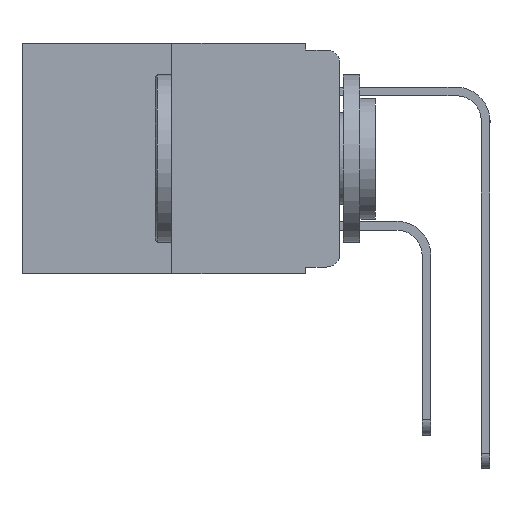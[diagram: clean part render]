
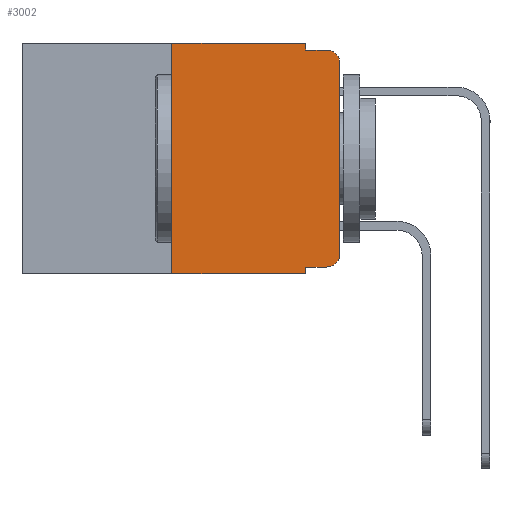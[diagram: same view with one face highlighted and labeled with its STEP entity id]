
A CAD part, left-side view. The second image highlights one B-rep face of the part: STEP entity #3002.
In plain terms, the highlighted planar face has unit normal (-1, 0, 0).
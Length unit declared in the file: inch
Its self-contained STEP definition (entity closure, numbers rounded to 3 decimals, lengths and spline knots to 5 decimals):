
#297 = EDGE_CURVE ( 'NONE', #541, #1149, #525, .T. ) ;
#336 = LINE ( 'NONE', #15332, #4701 ) ;
#396 = ORIENTED_EDGE ( 'NONE', *, *, #9617, .F. ) ;
#525 = LINE ( 'NONE', #19339, #12760 ) ;
#541 = VERTEX_POINT ( 'NONE', #13441 ) ;
#1149 = VERTEX_POINT ( 'NONE', #13604 ) ;
#1391 = VERTEX_POINT ( 'NONE', #6927 ) ;
#1458 = ORIENTED_EDGE ( 'NONE', *, *, #6786, .F. ) ;
#1470 = VERTEX_POINT ( 'NONE', #7637 ) ;
#1558 = LINE ( 'NONE', #17015, #4329 ) ;
#1567 = VERTEX_POINT ( 'NONE', #2991 ) ;
#1580 = DIRECTION ( 'NONE',  ( 0., 0., -1. ) ) ;
#1585 = DIRECTION ( 'NONE',  ( -1., 0., 0. ) ) ;
#1731 = LINE ( 'NONE', #12327, #9806 ) ;
#1735 = CARTESIAN_POINT ( 'NONE',  ( 0., 0.02, -0.03 ) ) ;
#2250 = CARTESIAN_POINT ( 'NONE',  ( 0., 0.051, -0.01 ) ) ;
#2991 = CARTESIAN_POINT ( 'NONE',  ( 0., 0.051, -0.343 ) ) ;
#3002 = ADVANCED_FACE ( 'NONE', ( #5109 ), #8063, .F. ) ;
#3426 = CARTESIAN_POINT ( 'NONE',  ( 0., 0.02, -0.313 ) ) ;
#3467 = ORIENTED_EDGE ( 'NONE', *, *, #17407, .F. ) ;
#3542 = CARTESIAN_POINT ( 'NONE',  ( 0., 0.02, -0.01 ) ) ;
#3921 = EDGE_CURVE ( 'NONE', #1391, #6474, #5566, .T. ) ;
#4329 = VECTOR ( 'NONE', #20122, 39.37008 ) ;
#4465 = CARTESIAN_POINT ( 'NONE',  ( 0., 0.02, -0.333 ) ) ;
#4498 = ORIENTED_EDGE ( 'NONE', *, *, #11927, .F. ) ;
#4673 = CIRCLE ( 'NONE', #9101, 0.02 ) ;
#4701 = VECTOR ( 'NONE', #6015, 39.37008 ) ;
#4958 = VECTOR ( 'NONE', #9388, 39.37008 ) ;
#5074 = DIRECTION ( 'NONE',  ( 0., 0., -1. ) ) ;
#5109 = FACE_OUTER_BOUND ( 'NONE', #13820, .T. ) ;
#5357 = CARTESIAN_POINT ( 'NONE',  ( 0., 0., -0.313 ) ) ;
#5566 = CIRCLE ( 'NONE', #9823, 0.02 ) ;
#5815 = VERTEX_POINT ( 'NONE', #14480 ) ;
#6015 = DIRECTION ( 'NONE',  ( 0., 0., -1. ) ) ;
#6028 = ORIENTED_EDGE ( 'NONE', *, *, #18913, .T. ) ;
#6474 = VERTEX_POINT ( 'NONE', #3542 ) ;
#6740 = DIRECTION ( 'NONE',  ( 0., 0., -1. ) ) ;
#6761 = DIRECTION ( 'NONE',  ( 1., 0., 0. ) ) ;
#6786 = EDGE_CURVE ( 'NONE', #1149, #5815, #8750, .T. ) ;
#6927 = CARTESIAN_POINT ( 'NONE',  ( 0., 0., -0.03 ) ) ;
#7637 = CARTESIAN_POINT ( 'NONE',  ( 0., 0.051, -0.333 ) ) ;
#7797 = ORIENTED_EDGE ( 'NONE', *, *, #12364, .T. ) ;
#7957 = CARTESIAN_POINT ( 'NONE',  ( 0., 0.473, 0. ) ) ;
#8063 = PLANE ( 'NONE',  #14039 ) ;
#8750 = LINE ( 'NONE', #9354, #4958 ) ;
#9101 = AXIS2_PLACEMENT_3D ( 'NONE', #3426, #14441, #5074 ) ;
#9354 = CARTESIAN_POINT ( 'NONE',  ( 0., 0.051, 0. ) ) ;
#9388 = DIRECTION ( 'NONE',  ( 0., 0., -1. ) ) ;
#9617 = EDGE_CURVE ( 'NONE', #5815, #6474, #14612, .T. ) ;
#9806 = VECTOR ( 'NONE', #13849, 39.37008 ) ;
#9823 = AXIS2_PLACEMENT_3D ( 'NONE', #1735, #1585, #1580 ) ;
#10190 = CARTESIAN_POINT ( 'NONE',  ( 0., 0.473, -0.343 ) ) ;
#10750 = ORIENTED_EDGE ( 'NONE', *, *, #15227, .T. ) ;
#11448 = VERTEX_POINT ( 'NONE', #4465 ) ;
#11927 = EDGE_CURVE ( 'NONE', #1470, #1567, #336, .T. ) ;
#12162 = ORIENTED_EDGE ( 'NONE', *, *, #14460, .T. ) ;
#12327 = CARTESIAN_POINT ( 'NONE',  ( 0., 0.051, -0.333 ) ) ;
#12335 = VERTEX_POINT ( 'NONE', #5357 ) ;
#12364 = EDGE_CURVE ( 'NONE', #18780, #1567, #17575, .T. ) ;
#12677 = DIRECTION ( 'NONE',  ( 0., 0., 1. ) ) ;
#12760 = VECTOR ( 'NONE', #19252, 39.37008 ) ;
#13189 = VECTOR ( 'NONE', #17928, 39.37008 ) ;
#13441 = CARTESIAN_POINT ( 'NONE',  ( 0., 0.25, 0. ) ) ;
#13525 = CARTESIAN_POINT ( 'NONE',  ( 0., 0.25, -0.343 ) ) ;
#13604 = CARTESIAN_POINT ( 'NONE',  ( 0., 0.051, 0. ) ) ;
#13820 = EDGE_LOOP ( 'NONE', ( #12162, #16705, #396, #1458, #19065, #3467, #7797, #4498, #6028, #10750 ) ) ;
#13849 = DIRECTION ( 'NONE',  ( 0., -1., 0. ) ) ;
#14039 = AXIS2_PLACEMENT_3D ( 'NONE', #7957, #6761, #6740 ) ;
#14441 = DIRECTION ( 'NONE',  ( -1., 0., 0. ) ) ;
#14460 = EDGE_CURVE ( 'NONE', #12335, #1391, #18706, .T. ) ;
#14480 = CARTESIAN_POINT ( 'NONE',  ( 0., 0.051, -0.01 ) ) ;
#14612 = LINE ( 'NONE', #2250, #13189 ) ;
#14660 = VECTOR ( 'NONE', #12677, 39.37008 ) ;
#14781 = DIRECTION ( 'NONE',  ( 0., -1., 0. ) ) ;
#15227 = EDGE_CURVE ( 'NONE', #11448, #12335, #4673, .T. ) ;
#15332 = CARTESIAN_POINT ( 'NONE',  ( 0., 0.051, 0. ) ) ;
#16633 = VECTOR ( 'NONE', #14781, 39.37008 ) ;
#16705 = ORIENTED_EDGE ( 'NONE', *, *, #3921, .T. ) ;
#17015 = CARTESIAN_POINT ( 'NONE',  ( 0., 0.25, 0. ) ) ;
#17407 = EDGE_CURVE ( 'NONE', #18780, #541, #1558, .T. ) ;
#17575 = LINE ( 'NONE', #10190, #16633 ) ;
#17928 = DIRECTION ( 'NONE',  ( 0., -1., 0. ) ) ;
#18706 = LINE ( 'NONE', #18731, #14660 ) ;
#18731 = CARTESIAN_POINT ( 'NONE',  ( 0., 0., 0. ) ) ;
#18780 = VERTEX_POINT ( 'NONE', #13525 ) ;
#18913 = EDGE_CURVE ( 'NONE', #1470, #11448, #1731, .T. ) ;
#19065 = ORIENTED_EDGE ( 'NONE', *, *, #297, .F. ) ;
#19252 = DIRECTION ( 'NONE',  ( 0., -1., 0. ) ) ;
#19339 = CARTESIAN_POINT ( 'NONE',  ( 0., 0.473, 0. ) ) ;
#20122 = DIRECTION ( 'NONE',  ( 0., 0., 1. ) ) ;
